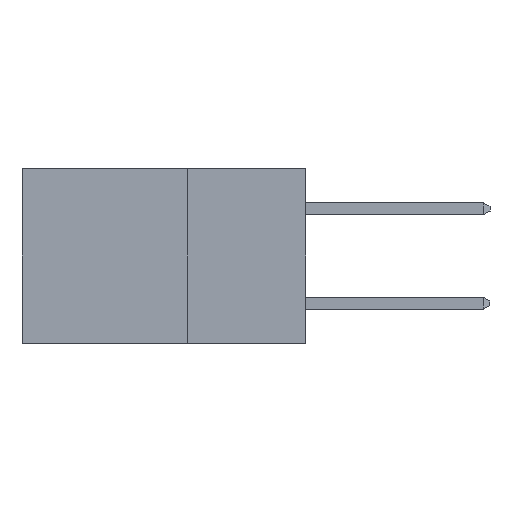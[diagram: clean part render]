
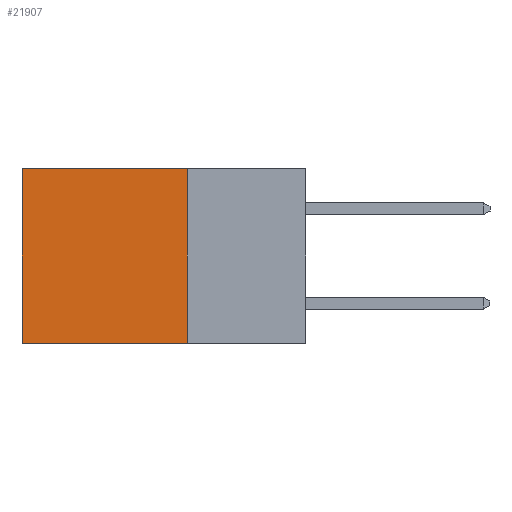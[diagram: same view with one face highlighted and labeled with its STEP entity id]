
A CAD part, left-side view. The second image highlights one B-rep face of the part: STEP entity #21907.
In plain terms, the highlighted planar face has unit normal (-1, 0, 0).
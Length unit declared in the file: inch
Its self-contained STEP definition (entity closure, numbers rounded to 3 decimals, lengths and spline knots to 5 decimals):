
#2149 = CARTESIAN_POINT ( 'NONE',  ( 0.298, 0.6, 0. ) ) ;
#2688 = PLANE ( 'NONE',  #28228 ) ;
#2970 = VERTEX_POINT ( 'NONE', #24356 ) ;
#3081 = EDGE_CURVE ( 'NONE', #7582, #2970, #11820, .T. ) ;
#4529 = VERTEX_POINT ( 'NONE', #24451 ) ;
#4925 = DIRECTION ( 'NONE',  ( 0., 0., -1. ) ) ;
#5990 = EDGE_CURVE ( 'NONE', #4529, #7582, #15216, .T. ) ;
#6096 = ORIENTED_EDGE ( 'NONE', *, *, #22569, .T. ) ;
#7169 = CARTESIAN_POINT ( 'NONE',  ( 0.298, 0.25, 0. ) ) ;
#7582 = VERTEX_POINT ( 'NONE', #15691 ) ;
#8818 = CARTESIAN_POINT ( 'NONE',  ( 0.298, 0.25, -0.37 ) ) ;
#9169 = DIRECTION ( 'NONE',  ( 0., 1., 0. ) ) ;
#9205 = VECTOR ( 'NONE', #12503, 39.37008 ) ;
#11622 = DIRECTION ( 'NONE',  ( 1., 0., 0. ) ) ;
#11820 = LINE ( 'NONE', #8818, #23611 ) ;
#12503 = DIRECTION ( 'NONE',  ( 0., 1., 0. ) ) ;
#13946 = EDGE_LOOP ( 'NONE', ( #6096, #23203, #17766, #15719 ) ) ;
#14290 = CARTESIAN_POINT ( 'NONE',  ( 0.298, 0.6, 0. ) ) ;
#15216 = LINE ( 'NONE', #24784, #22177 ) ;
#15470 = LINE ( 'NONE', #14290, #26572 ) ;
#15691 = CARTESIAN_POINT ( 'NONE',  ( 0.298, 0.25, -0.37 ) ) ;
#15719 = ORIENTED_EDGE ( 'NONE', *, *, #23252, .T. ) ;
#16487 = DIRECTION ( 'NONE',  ( 0., 0., -1. ) ) ;
#17766 = ORIENTED_EDGE ( 'NONE', *, *, #5990, .F. ) ;
#19210 = CARTESIAN_POINT ( 'NONE',  ( 0.298, 0.25, 0. ) ) ;
#20297 = LINE ( 'NONE', #19210, #9205 ) ;
#21907 = ADVANCED_FACE ( 'NONE', ( #27642 ), #2688, .F. ) ;
#22177 = VECTOR ( 'NONE', #4925, 39.37008 ) ;
#22569 = EDGE_CURVE ( 'NONE', #25982, #2970, #15470, .T. ) ;
#23203 = ORIENTED_EDGE ( 'NONE', *, *, #3081, .F. ) ;
#23252 = EDGE_CURVE ( 'NONE', #4529, #25982, #20297, .T. ) ;
#23611 = VECTOR ( 'NONE', #9169, 39.37008 ) ;
#24356 = CARTESIAN_POINT ( 'NONE',  ( 0.298, 0.6, -0.37 ) ) ;
#24451 = CARTESIAN_POINT ( 'NONE',  ( 0.298, 0.25, 0. ) ) ;
#24784 = CARTESIAN_POINT ( 'NONE',  ( 0.298, 0.25, 0. ) ) ;
#25982 = VERTEX_POINT ( 'NONE', #2149 ) ;
#26572 = VECTOR ( 'NONE', #16487, 39.37008 ) ;
#27108 = DIRECTION ( 'NONE',  ( 0., 0., -1. ) ) ;
#27642 = FACE_OUTER_BOUND ( 'NONE', #13946, .T. ) ;
#28228 = AXIS2_PLACEMENT_3D ( 'NONE', #7169, #11622, #27108 ) ;
